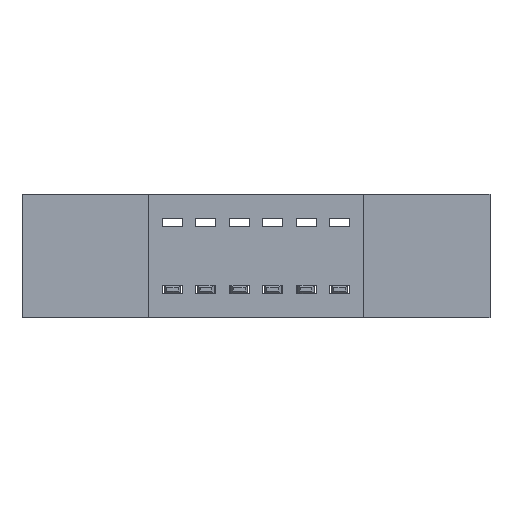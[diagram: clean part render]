
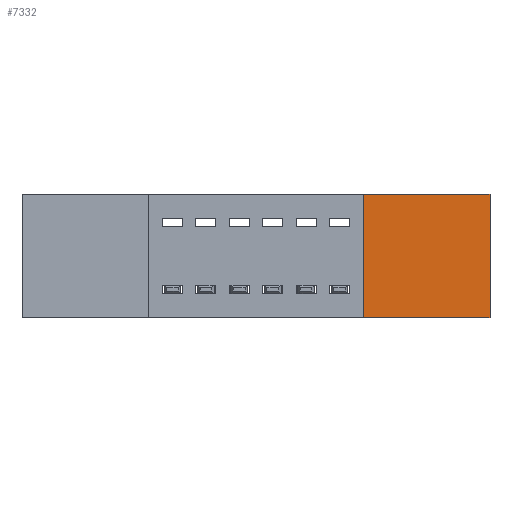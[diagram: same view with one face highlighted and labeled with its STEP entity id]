
A CAD part, front view. The second image highlights one B-rep face of the part: STEP entity #7332.
In plain terms, the highlighted planar face has unit normal (0, -1, 0).
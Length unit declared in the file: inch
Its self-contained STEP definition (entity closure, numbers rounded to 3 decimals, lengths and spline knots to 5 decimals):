
#19 = PLANE ( 'NONE',  #2306 ) ;
#301 = LINE ( 'NONE', #922, #3508 ) ;
#305 = DIRECTION ( 'NONE',  ( 1., 0., 0. ) ) ;
#423 = DIRECTION ( 'NONE',  ( 0., 0., 1. ) ) ;
#595 = VECTOR ( 'NONE', #305, 39.37008 ) ;
#643 = DIRECTION ( 'NONE',  ( 0., -1., 0. ) ) ;
#922 = CARTESIAN_POINT ( 'NONE',  ( 1.023, 0., -0.37 ) ) ;
#1030 = DIRECTION ( 'NONE',  ( -1., 0., 0. ) ) ;
#1831 = EDGE_CURVE ( 'NONE', #4329, #3694, #7229, .T. ) ;
#2156 = CARTESIAN_POINT ( 'NONE',  ( 0., 0., 0. ) ) ;
#2306 = AXIS2_PLACEMENT_3D ( 'NONE', #7980, #643, #7935 ) ;
#3323 = EDGE_CURVE ( 'NONE', #4430, #5997, #301, .T. ) ;
#3508 = VECTOR ( 'NONE', #423, 39.37008 ) ;
#3694 = VERTEX_POINT ( 'NONE', #5807 ) ;
#3722 = VECTOR ( 'NONE', #4913, 39.37008 ) ;
#3861 = LINE ( 'NONE', #4682, #6472 ) ;
#4207 = CARTESIAN_POINT ( 'NONE',  ( 1.023, 0., 0. ) ) ;
#4329 = VERTEX_POINT ( 'NONE', #4596 ) ;
#4430 = VERTEX_POINT ( 'NONE', #5299 ) ;
#4518 = ORIENTED_EDGE ( 'NONE', *, *, #7941, .F. ) ;
#4596 = CARTESIAN_POINT ( 'NONE',  ( 1.4, 0., 0. ) ) ;
#4682 = CARTESIAN_POINT ( 'NONE',  ( 0., 0., -0.37 ) ) ;
#4913 = DIRECTION ( 'NONE',  ( 0., 0., -1. ) ) ;
#5094 = ORIENTED_EDGE ( 'NONE', *, *, #3323, .F. ) ;
#5299 = CARTESIAN_POINT ( 'NONE',  ( 1.023, 0., -0.37 ) ) ;
#5638 = FACE_OUTER_BOUND ( 'NONE', #7267, .T. ) ;
#5725 = LINE ( 'NONE', #2156, #595 ) ;
#5807 = CARTESIAN_POINT ( 'NONE',  ( 1.4, 0., -0.37 ) ) ;
#5997 = VERTEX_POINT ( 'NONE', #4207 ) ;
#6472 = VECTOR ( 'NONE', #1030, 39.37008 ) ;
#6485 = ORIENTED_EDGE ( 'NONE', *, *, #1831, .F. ) ;
#7229 = LINE ( 'NONE', #7755, #3722 ) ;
#7267 = EDGE_LOOP ( 'NONE', ( #5094, #7766, #6485, #4518 ) ) ;
#7332 = ADVANCED_FACE ( 'NONE', ( #5638 ), #19, .T. ) ;
#7410 = EDGE_CURVE ( 'NONE', #3694, #4430, #3861, .T. ) ;
#7755 = CARTESIAN_POINT ( 'NONE',  ( 1.4, 0., 0. ) ) ;
#7766 = ORIENTED_EDGE ( 'NONE', *, *, #7410, .F. ) ;
#7935 = DIRECTION ( 'NONE',  ( 0., 0., -1. ) ) ;
#7941 = EDGE_CURVE ( 'NONE', #5997, #4329, #5725, .T. ) ;
#7980 = CARTESIAN_POINT ( 'NONE',  ( 0., 0., -0.37 ) ) ;
